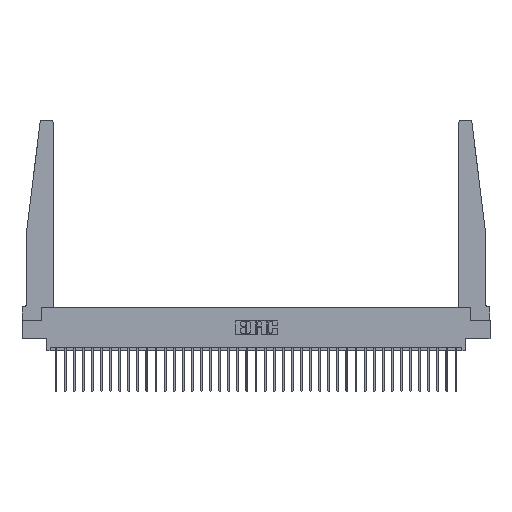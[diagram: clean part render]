
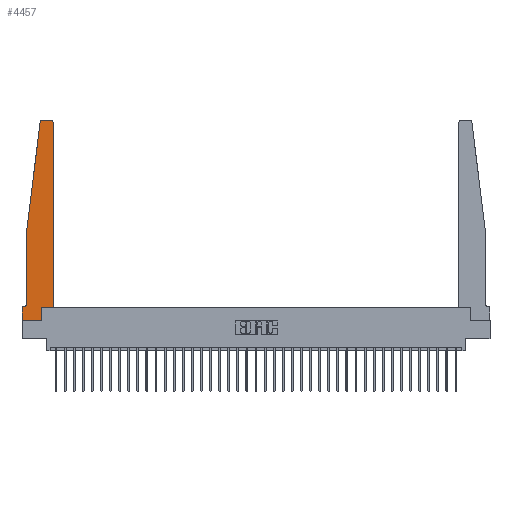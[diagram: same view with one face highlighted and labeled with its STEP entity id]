
A CAD part, top view. The second image highlights one B-rep face of the part: STEP entity #4457.
In plain terms, the highlighted planar face has unit normal (0, 0, 1).
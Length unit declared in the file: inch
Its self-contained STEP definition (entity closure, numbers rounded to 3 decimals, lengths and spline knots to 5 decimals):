
#81 = VERTEX_POINT ( 'NONE', #14633 ) ;
#704 = EDGE_CURVE ( 'NONE', #19819, #26127, #2680, .T. ) ;
#1007 = VECTOR ( 'NONE', #22144, 39.37008 ) ;
#1258 = VECTOR ( 'NONE', #8013, 39.37008 ) ;
#1439 = VERTEX_POINT ( 'NONE', #20713 ) ;
#1586 = CARTESIAN_POINT ( 'NONE',  ( 0.2605, 0.18, 0.37 ) ) ;
#1673 = LINE ( 'NONE', #13637, #21794 ) ;
#2116 = LINE ( 'NONE', #28928, #1258 ) ;
#2329 = VERTEX_POINT ( 'NONE', #13856 ) ;
#2391 = LINE ( 'NONE', #26387, #15537 ) ;
#2474 = DIRECTION ( 'NONE',  ( -1., 0., 0. ) ) ;
#2680 = LINE ( 'NONE', #9092, #1007 ) ;
#2705 = LINE ( 'NONE', #31964, #9700 ) ;
#3220 = CARTESIAN_POINT ( 'NONE',  ( 0.27653, 2.72, 0.37 ) ) ;
#3245 = FACE_OUTER_BOUND ( 'NONE', #5028, .T. ) ;
#3579 = ORIENTED_EDGE ( 'NONE', *, *, #6687, .T. ) ;
#3715 = EDGE_CURVE ( 'NONE', #17009, #18602, #7843, .T. ) ;
#3895 = EDGE_CURVE ( 'NONE', #18602, #7718, #18837, .T. ) ;
#4457 = ADVANCED_FACE ( 'NONE', ( #3245 ), #16797, .T. ) ;
#4841 = CARTESIAN_POINT ( 'NONE',  ( 0.27653, 2.75, 0.37 ) ) ;
#5028 = EDGE_LOOP ( 'NONE', ( #3579, #5247, #6890, #27738, #8527, #22449, #23272, #17108, #24082, #17917, #19559, #15105 ) ) ;
#5247 = ORIENTED_EDGE ( 'NONE', *, *, #32848, .T. ) ;
#5887 = DIRECTION ( 'NONE',  ( 1., 0., 0. ) ) ;
#6687 = EDGE_CURVE ( 'NONE', #7718, #17259, #9535, .T. ) ;
#6890 = ORIENTED_EDGE ( 'NONE', *, *, #704, .T. ) ;
#6892 = CARTESIAN_POINT ( 'NONE',  ( 0.25, 2.75, 0.37 ) ) ;
#6942 = EDGE_CURVE ( 'NONE', #12811, #2329, #2116, .T. ) ;
#7362 = CARTESIAN_POINT ( 'NONE',  ( 0., 0., 0.37 ) ) ;
#7718 = VERTEX_POINT ( 'NONE', #26699 ) ;
#7843 = LINE ( 'NONE', #32284, #17626 ) ;
#8013 = DIRECTION ( 'NONE',  ( 1., 0., 0. ) ) ;
#8112 = VERTEX_POINT ( 'NONE', #22172 ) ;
#8114 = DIRECTION ( 'NONE',  ( 0., -1., 0. ) ) ;
#8527 = ORIENTED_EDGE ( 'NONE', *, *, #9626, .T. ) ;
#8574 = LINE ( 'NONE', #33296, #15540 ) ;
#9092 = CARTESIAN_POINT ( 'NONE',  ( 0.065, 1.25, 0.37 ) ) ;
#9400 = DIRECTION ( 'NONE',  ( -1., 0., 0. ) ) ;
#9535 = LINE ( 'NONE', #6892, #29585 ) ;
#9626 = EDGE_CURVE ( 'NONE', #8112, #1439, #31882, .T. ) ;
#9700 = VECTOR ( 'NONE', #16297, 39.37008 ) ;
#9750 = EDGE_CURVE ( 'NONE', #81, #12811, #2391, .T. ) ;
#10843 = VERTEX_POINT ( 'NONE', #1586 ) ;
#12811 = VERTEX_POINT ( 'NONE', #7362 ) ;
#13637 = CARTESIAN_POINT ( 'NONE',  ( 0.425, 0.18, 0.37 ) ) ;
#13856 = CARTESIAN_POINT ( 'NONE',  ( 0.2605, 0., 0.37 ) ) ;
#14364 = CARTESIAN_POINT ( 'NONE',  ( 0.425, 0.18, 0.37 ) ) ;
#14633 = CARTESIAN_POINT ( 'NONE',  ( 0., 0.1875, 0.37 ) ) ;
#14689 = DIRECTION ( 'NONE',  ( 0., 0., 1. ) ) ;
#14819 = EDGE_CURVE ( 'NONE', #2329, #10843, #8574, .T. ) ;
#15044 = DIRECTION ( 'NONE',  ( 0., 1., 0. ) ) ;
#15105 = ORIENTED_EDGE ( 'NONE', *, *, #3895, .T. ) ;
#15537 = VECTOR ( 'NONE', #8114, 39.37008 ) ;
#15540 = VECTOR ( 'NONE', #15044, 39.37008 ) ;
#16297 = DIRECTION ( 'NONE',  ( -1., 0., 0. ) ) ;
#16738 = AXIS2_PLACEMENT_3D ( 'NONE', #27319, #32572, #16908 ) ;
#16797 = PLANE ( 'NONE',  #16738 ) ;
#16908 = DIRECTION ( 'NONE',  ( 1., 0., 0. ) ) ;
#17009 = VERTEX_POINT ( 'NONE', #14364 ) ;
#17108 = ORIENTED_EDGE ( 'NONE', *, *, #6942, .T. ) ;
#17259 = VERTEX_POINT ( 'NONE', #4841 ) ;
#17626 = VECTOR ( 'NONE', #29660, 39.37008 ) ;
#17827 = EDGE_CURVE ( 'NONE', #26127, #8112, #30087, .T. ) ;
#17917 = ORIENTED_EDGE ( 'NONE', *, *, #22476, .T. ) ;
#18148 = DIRECTION ( 'NONE',  ( 0., 0., -1. ) ) ;
#18602 = VERTEX_POINT ( 'NONE', #23642 ) ;
#18747 = EDGE_CURVE ( 'NONE', #1439, #81, #2705, .T. ) ;
#18837 = CIRCLE ( 'NONE', #33810, 0.03 ) ;
#18869 = DIRECTION ( 'NONE',  ( 1., 0., 0. ) ) ;
#19559 = ORIENTED_EDGE ( 'NONE', *, *, #3715, .T. ) ;
#19819 = VERTEX_POINT ( 'NONE', #33368 ) ;
#20586 = CARTESIAN_POINT ( 'NONE',  ( 0.065, 1.25, 0.37 ) ) ;
#20713 = CARTESIAN_POINT ( 'NONE',  ( 0.015, 0.1875, 0.37 ) ) ;
#21553 = DIRECTION ( 'NONE',  ( 0., 0., 1. ) ) ;
#21794 = VECTOR ( 'NONE', #18869, 39.37008 ) ;
#22125 = AXIS2_PLACEMENT_3D ( 'NONE', #33838, #18148, #2474 ) ;
#22144 = DIRECTION ( 'NONE',  ( -0.122, -0.992, 0. ) ) ;
#22172 = CARTESIAN_POINT ( 'NONE',  ( 0.065, 0.2375, 0.37 ) ) ;
#22449 = ORIENTED_EDGE ( 'NONE', *, *, #18747, .T. ) ;
#22476 = EDGE_CURVE ( 'NONE', #10843, #17009, #1673, .T. ) ;
#23152 = VECTOR ( 'NONE', #23238, 39.37008 ) ;
#23238 = DIRECTION ( 'NONE',  ( 0., -1., 0. ) ) ;
#23272 = ORIENTED_EDGE ( 'NONE', *, *, #9750, .T. ) ;
#23642 = CARTESIAN_POINT ( 'NONE',  ( 0.425, 2.72, 0.37 ) ) ;
#24082 = ORIENTED_EDGE ( 'NONE', *, *, #14819, .T. ) ;
#24454 = CARTESIAN_POINT ( 'NONE',  ( 0.065, 1.25, 0.37 ) ) ;
#26127 = VERTEX_POINT ( 'NONE', #24454 ) ;
#26387 = CARTESIAN_POINT ( 'NONE',  ( 0., 0., 0.37 ) ) ;
#26699 = CARTESIAN_POINT ( 'NONE',  ( 0.395, 2.75, 0.37 ) ) ;
#27165 = CIRCLE ( 'NONE', #28884, 0.03 ) ;
#27319 = CARTESIAN_POINT ( 'NONE',  ( 0., 0.1875, 0.37 ) ) ;
#27738 = ORIENTED_EDGE ( 'NONE', *, *, #17827, .T. ) ;
#28884 = AXIS2_PLACEMENT_3D ( 'NONE', #3220, #21553, #5887 ) ;
#28928 = CARTESIAN_POINT ( 'NONE',  ( 0., 0., 0.37 ) ) ;
#29585 = VECTOR ( 'NONE', #9400, 39.37008 ) ;
#29660 = DIRECTION ( 'NONE',  ( 0., 1., 0. ) ) ;
#30087 = LINE ( 'NONE', #20586, #23152 ) ;
#30325 = CARTESIAN_POINT ( 'NONE',  ( 0.395, 2.72, 0.37 ) ) ;
#31882 = CIRCLE ( 'NONE', #22125, 0.05 ) ;
#31964 = CARTESIAN_POINT ( 'NONE',  ( 0.065, 0.1875, 0.37 ) ) ;
#32284 = CARTESIAN_POINT ( 'NONE',  ( 0.425, 0.18, 0.37 ) ) ;
#32572 = DIRECTION ( 'NONE',  ( 0., 0., 1. ) ) ;
#32848 = EDGE_CURVE ( 'NONE', #17259, #19819, #27165, .T. ) ;
#32939 = DIRECTION ( 'NONE',  ( 1., 0., 0. ) ) ;
#33296 = CARTESIAN_POINT ( 'NONE',  ( 0.2605, 0.18, 0.37 ) ) ;
#33368 = CARTESIAN_POINT ( 'NONE',  ( 0.24675, 2.72367, 0.37 ) ) ;
#33810 = AXIS2_PLACEMENT_3D ( 'NONE', #30325, #14689, #32939 ) ;
#33838 = CARTESIAN_POINT ( 'NONE',  ( 0.015, 0.2375, 0.37 ) ) ;
